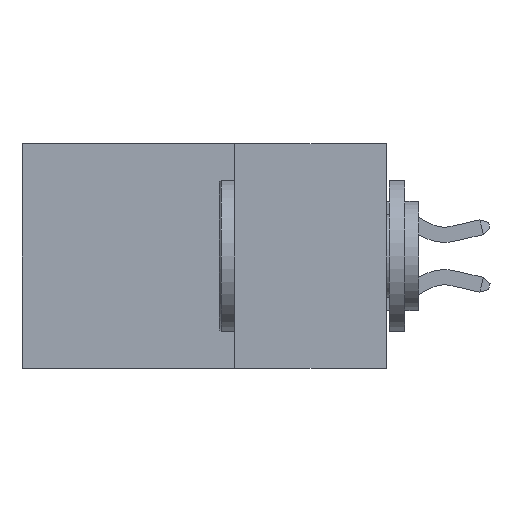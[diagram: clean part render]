
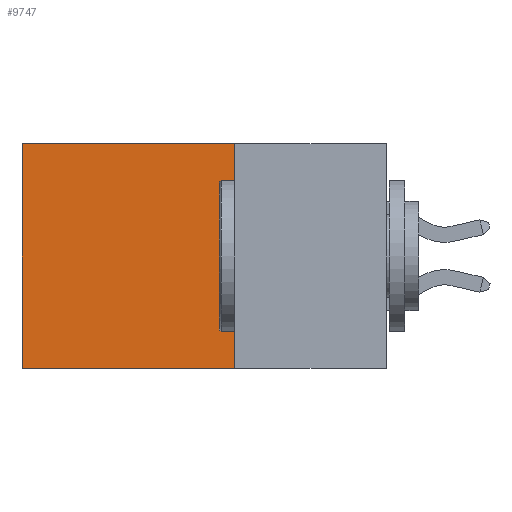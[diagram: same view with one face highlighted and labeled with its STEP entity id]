
A CAD part, left-side view. The second image highlights one B-rep face of the part: STEP entity #9747.
In plain terms, the highlighted planar face has unit normal (-1, 0, 0).
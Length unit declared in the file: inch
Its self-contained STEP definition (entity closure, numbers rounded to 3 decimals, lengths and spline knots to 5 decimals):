
#198 = CARTESIAN_POINT ( 'NONE',  ( 0.2615, 0.6, -0.37 ) ) ;
#329 = LINE ( 'NONE', #17840, #16123 ) ;
#663 = VERTEX_POINT ( 'NONE', #24100 ) ;
#2271 = EDGE_CURVE ( 'NONE', #20571, #19688, #329, .T. ) ;
#3212 = CARTESIAN_POINT ( 'NONE',  ( 0.2615, 0.25, -0.37 ) ) ;
#3398 = VERTEX_POINT ( 'NONE', #7037 ) ;
#3581 = DIRECTION ( 'NONE',  ( 0., 0., -1. ) ) ;
#3792 = CARTESIAN_POINT ( 'NONE',  ( 0.2615, 0.25, -0.37 ) ) ;
#5082 = EDGE_LOOP ( 'NONE', ( #9011, #18235, #20435, #15379 ) ) ;
#5878 = DIRECTION ( 'NONE',  ( 0., 0., -1. ) ) ;
#6208 = DIRECTION ( 'NONE',  ( 0., 1., 0. ) ) ;
#7037 = CARTESIAN_POINT ( 'NONE',  ( 0.2615, 0.6, 0. ) ) ;
#8320 = VECTOR ( 'NONE', #10646, 39.37008 ) ;
#8682 = CARTESIAN_POINT ( 'NONE',  ( 0.2615, 0.6, -0.37 ) ) ;
#8972 = LINE ( 'NONE', #198, #8320 ) ;
#9011 = ORIENTED_EDGE ( 'NONE', *, *, #23077, .T. ) ;
#9747 = ADVANCED_FACE ( 'NONE', ( #24461 ), #19945, .F. ) ;
#10646 = DIRECTION ( 'NONE',  ( 0., 0., -1. ) ) ;
#13453 = VECTOR ( 'NONE', #21458, 39.37008 ) ;
#13498 = CARTESIAN_POINT ( 'NONE',  ( 0.2615, 0.25, 0. ) ) ;
#15379 = ORIENTED_EDGE ( 'NONE', *, *, #21217, .T. ) ;
#15877 = EDGE_CURVE ( 'NONE', #663, #20571, #22183, .T. ) ;
#16123 = VECTOR ( 'NONE', #6208, 39.37008 ) ;
#17840 = CARTESIAN_POINT ( 'NONE',  ( 0.2615, 0.25, -0.37 ) ) ;
#18049 = DIRECTION ( 'NONE',  ( 1., 0., 0. ) ) ;
#18199 = LINE ( 'NONE', #13498, #13453 ) ;
#18235 = ORIENTED_EDGE ( 'NONE', *, *, #2271, .F. ) ;
#19688 = VERTEX_POINT ( 'NONE', #8682 ) ;
#19762 = CARTESIAN_POINT ( 'NONE',  ( 0.2615, 0.25, -0.37 ) ) ;
#19831 = AXIS2_PLACEMENT_3D ( 'NONE', #3792, #18049, #5878 ) ;
#19945 = PLANE ( 'NONE',  #19831 ) ;
#20435 = ORIENTED_EDGE ( 'NONE', *, *, #15877, .F. ) ;
#20571 = VERTEX_POINT ( 'NONE', #3212 ) ;
#21217 = EDGE_CURVE ( 'NONE', #663, #3398, #18199, .T. ) ;
#21458 = DIRECTION ( 'NONE',  ( 0., 1., 0. ) ) ;
#21544 = VECTOR ( 'NONE', #3581, 39.37008 ) ;
#22183 = LINE ( 'NONE', #19762, #21544 ) ;
#23077 = EDGE_CURVE ( 'NONE', #3398, #19688, #8972, .T. ) ;
#24100 = CARTESIAN_POINT ( 'NONE',  ( 0.2615, 0.25, 0. ) ) ;
#24461 = FACE_OUTER_BOUND ( 'NONE', #5082, .T. ) ;
